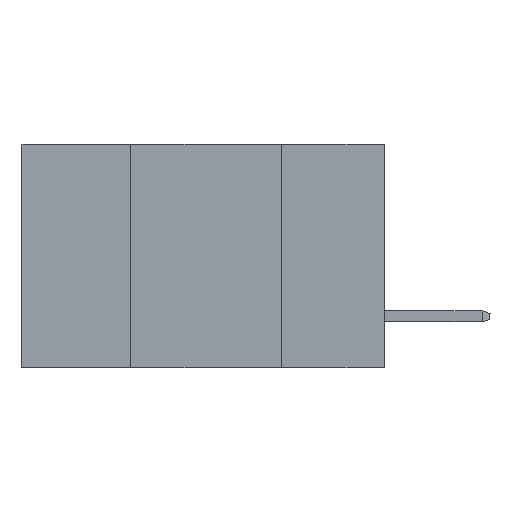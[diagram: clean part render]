
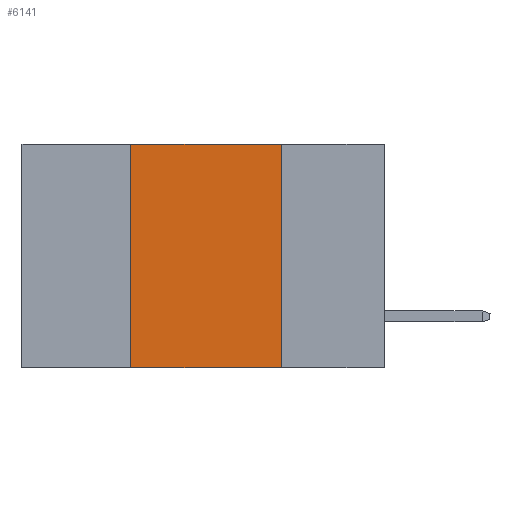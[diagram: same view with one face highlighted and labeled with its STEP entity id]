
A CAD part, left-side view. The second image highlights one B-rep face of the part: STEP entity #6141.
In plain terms, the highlighted planar face has unit normal (-1, 0, 0).
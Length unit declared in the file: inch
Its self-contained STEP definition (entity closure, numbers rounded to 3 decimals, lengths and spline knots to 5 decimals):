
#542 = DIRECTION ( 'NONE',  ( 0., 0., -1. ) ) ;
#1144 = VECTOR ( 'NONE', #8166, 39.37008 ) ;
#1843 = ORIENTED_EDGE ( 'NONE', *, *, #15090, .F. ) ;
#1855 = VERTEX_POINT ( 'NONE', #13643 ) ;
#2626 = ORIENTED_EDGE ( 'NONE', *, *, #10422, .F. ) ;
#2968 = DIRECTION ( 'NONE',  ( 0., -1., 0. ) ) ;
#3317 = LINE ( 'NONE', #16915, #9796 ) ;
#4610 = ORIENTED_EDGE ( 'NONE', *, *, #16175, .F. ) ;
#4670 = ORIENTED_EDGE ( 'NONE', *, *, #15922, .T. ) ;
#6141 = ADVANCED_FACE ( 'NONE', ( #17522 ), #7670, .F. ) ;
#7363 = CARTESIAN_POINT ( 'NONE',  ( 0., 0.42, 0. ) ) ;
#7453 = AXIS2_PLACEMENT_3D ( 'NONE', #14719, #13303, #542 ) ;
#7670 = PLANE ( 'NONE',  #7453 ) ;
#7868 = VECTOR ( 'NONE', #11875, 39.37008 ) ;
#8166 = DIRECTION ( 'NONE',  ( 0., -1., 0. ) ) ;
#9410 = CARTESIAN_POINT ( 'NONE',  ( 0., 0.17, 0. ) ) ;
#9516 = CARTESIAN_POINT ( 'NONE',  ( 0., 0.6, -0.37 ) ) ;
#9796 = VECTOR ( 'NONE', #2968, 39.37008 ) ;
#9973 = VERTEX_POINT ( 'NONE', #11403 ) ;
#10422 = EDGE_CURVE ( 'NONE', #9973, #16996, #3317, .T. ) ;
#10884 = DIRECTION ( 'NONE',  ( 0., 0., -1. ) ) ;
#11403 = CARTESIAN_POINT ( 'NONE',  ( 0., 0.42, 0. ) ) ;
#11670 = LINE ( 'NONE', #7363, #7868 ) ;
#11875 = DIRECTION ( 'NONE',  ( 0., 0., 1. ) ) ;
#12045 = CARTESIAN_POINT ( 'NONE',  ( 0., 0.17, -0.37 ) ) ;
#13303 = DIRECTION ( 'NONE',  ( 1., 0., 0. ) ) ;
#13643 = CARTESIAN_POINT ( 'NONE',  ( 0., 0.42, -0.37 ) ) ;
#13832 = CARTESIAN_POINT ( 'NONE',  ( 0., 0.17, 0. ) ) ;
#14108 = LINE ( 'NONE', #9410, #14507 ) ;
#14507 = VECTOR ( 'NONE', #10884, 39.37008 ) ;
#14719 = CARTESIAN_POINT ( 'NONE',  ( 0., 0.6, 0. ) ) ;
#15090 = EDGE_CURVE ( 'NONE', #1855, #9973, #11670, .T. ) ;
#15922 = EDGE_CURVE ( 'NONE', #1855, #18074, #16055, .T. ) ;
#16055 = LINE ( 'NONE', #9516, #1144 ) ;
#16175 = EDGE_CURVE ( 'NONE', #16996, #18074, #14108, .T. ) ;
#16915 = CARTESIAN_POINT ( 'NONE',  ( 0., 0.6, 0. ) ) ;
#16996 = VERTEX_POINT ( 'NONE', #13832 ) ;
#17522 = FACE_OUTER_BOUND ( 'NONE', #17607, .T. ) ;
#17607 = EDGE_LOOP ( 'NONE', ( #4610, #2626, #1843, #4670 ) ) ;
#18074 = VERTEX_POINT ( 'NONE', #12045 ) ;
